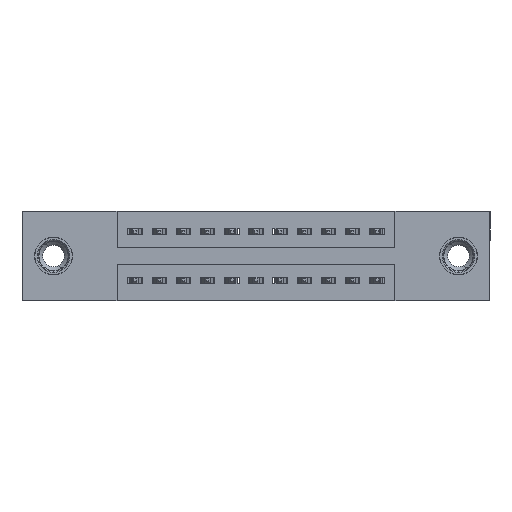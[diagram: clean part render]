
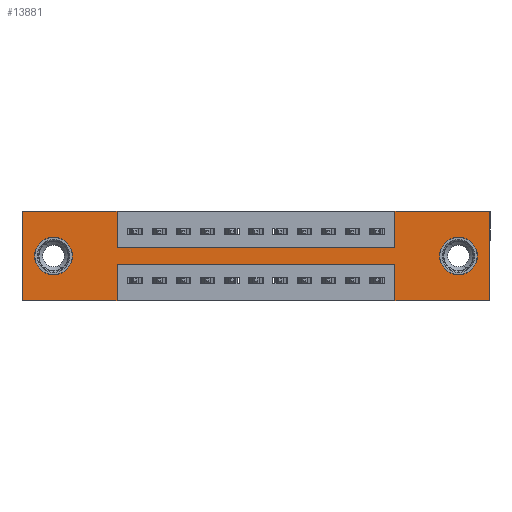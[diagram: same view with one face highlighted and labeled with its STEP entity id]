
A CAD part, front view. The second image highlights one B-rep face of the part: STEP entity #13881.
In plain terms, the highlighted planar face has unit normal (0, -1, 0).
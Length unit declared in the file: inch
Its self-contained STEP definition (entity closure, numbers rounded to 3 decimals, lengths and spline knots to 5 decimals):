
#4 = DIRECTION ( 'NONE',  ( 0., 0., -1. ) ) ;
#29 = CARTESIAN_POINT ( 'NONE',  ( 1.5425, 0., 0. ) ) ;
#186 = EDGE_CURVE ( 'NONE', #11152, #595, #14252, .T. ) ;
#595 = VERTEX_POINT ( 'NONE', #15899 ) ;
#646 = CIRCLE ( 'NONE', #2475, 0.078 ) ;
#793 = AXIS2_PLACEMENT_3D ( 'NONE', #12753, #14285, #6076 ) ;
#917 = CIRCLE ( 'NONE', #13022, 0.078 ) ;
#1027 = ORIENTED_EDGE ( 'NONE', *, *, #2276, .F. ) ;
#1037 = CARTESIAN_POINT ( 'NONE',  ( 0., 0., -0.37 ) ) ;
#1091 = DIRECTION ( 'NONE',  ( 0., -1., 0. ) ) ;
#1112 = EDGE_CURVE ( 'NONE', #6410, #12176, #646, .T. ) ;
#1217 = VERTEX_POINT ( 'NONE', #5519 ) ;
#1307 = DIRECTION ( 'NONE',  ( -1., 0., 0. ) ) ;
#1494 = ORIENTED_EDGE ( 'NONE', *, *, #11015, .F. ) ;
#1873 = EDGE_CURVE ( 'NONE', #595, #14750, #13383, .T. ) ;
#1982 = CARTESIAN_POINT ( 'NONE',  ( 0., 0., -0.37 ) ) ;
#2038 = DIRECTION ( 'NONE',  ( 0., 1., 0. ) ) ;
#2178 = FACE_BOUND ( 'NONE', #6233, .T. ) ;
#2208 = VERTEX_POINT ( 'NONE', #7370 ) ;
#2276 = EDGE_CURVE ( 'NONE', #14750, #14485, #16325, .T. ) ;
#2378 = LINE ( 'NONE', #16224, #17463 ) ;
#2394 = EDGE_LOOP ( 'NONE', ( #10713, #16401 ) ) ;
#2475 = AXIS2_PLACEMENT_3D ( 'NONE', #17480, #9263, #9315 ) ;
#2486 = ORIENTED_EDGE ( 'NONE', *, *, #6051, .T. ) ;
#2535 = VECTOR ( 'NONE', #13410, 39.37008 ) ;
#2538 = CARTESIAN_POINT ( 'NONE',  ( 0., 0., -0.37 ) ) ;
#2643 = ORIENTED_EDGE ( 'NONE', *, *, #10460, .F. ) ;
#2704 = VECTOR ( 'NONE', #10745, 39.37008 ) ;
#3094 = LINE ( 'NONE', #14840, #7967 ) ;
#3532 = VERTEX_POINT ( 'NONE', #29 ) ;
#3795 = DIRECTION ( 'NONE',  ( 0., 0., -1. ) ) ;
#3907 = DIRECTION ( 'NONE',  ( 0., 0., -1. ) ) ;
#3909 = EDGE_CURVE ( 'NONE', #1217, #11836, #12257, .T. ) ;
#3942 = AXIS2_PLACEMENT_3D ( 'NONE', #1037, #1091, #3795 ) ;
#4038 = EDGE_CURVE ( 'NONE', #14485, #5997, #5833, .T. ) ;
#4094 = PLANE ( 'NONE',  #3942 ) ;
#4148 = CARTESIAN_POINT ( 'NONE',  ( 0.3925, 0., 0. ) ) ;
#4479 = DIRECTION ( 'NONE',  ( 1., 0., 0. ) ) ;
#4730 = ORIENTED_EDGE ( 'NONE', *, *, #4038, .F. ) ;
#4836 = LINE ( 'NONE', #4148, #9075 ) ;
#5200 = ORIENTED_EDGE ( 'NONE', *, *, #15772, .F. ) ;
#5343 = LINE ( 'NONE', #12643, #8520 ) ;
#5519 = CARTESIAN_POINT ( 'NONE',  ( 0.3925, 0., -0.37 ) ) ;
#5765 = FACE_BOUND ( 'NONE', #2394, .T. ) ;
#5833 = LINE ( 'NONE', #6760, #15400 ) ;
#5997 = VERTEX_POINT ( 'NONE', #7391 ) ;
#6051 = EDGE_CURVE ( 'NONE', #12176, #6410, #9373, .T. ) ;
#6076 = DIRECTION ( 'NONE',  ( 0., 0., -1. ) ) ;
#6093 = LINE ( 'NONE', #13523, #2704 ) ;
#6233 = EDGE_LOOP ( 'NONE', ( #2486, #9530 ) ) ;
#6410 = VERTEX_POINT ( 'NONE', #8038 ) ;
#6420 = EDGE_CURVE ( 'NONE', #9613, #2208, #917, .T. ) ;
#6482 = ORIENTED_EDGE ( 'NONE', *, *, #3909, .F. ) ;
#6563 = EDGE_CURVE ( 'NONE', #11707, #15622, #5343, .T. ) ;
#6593 = CARTESIAN_POINT ( 'NONE',  ( 1.5425, 0., -0.37 ) ) ;
#6622 = FACE_OUTER_BOUND ( 'NONE', #13004, .T. ) ;
#6669 = EDGE_CURVE ( 'NONE', #5997, #1217, #10465, .T. ) ;
#6712 = DIRECTION ( 'NONE',  ( 0., 0., 1. ) ) ;
#6760 = CARTESIAN_POINT ( 'NONE',  ( 0.3925, 0., -0.22 ) ) ;
#7326 = DIRECTION ( 'NONE',  ( 1., 0., 0. ) ) ;
#7370 = CARTESIAN_POINT ( 'NONE',  ( 1.805, 0., -0.263 ) ) ;
#7391 = CARTESIAN_POINT ( 'NONE',  ( 0.3925, 0., -0.22 ) ) ;
#7558 = ORIENTED_EDGE ( 'NONE', *, *, #186, .F. ) ;
#7594 = EDGE_CURVE ( 'NONE', #13691, #3532, #2378, .T. ) ;
#7871 = VERTEX_POINT ( 'NONE', #12721 ) ;
#7967 = VECTOR ( 'NONE', #12130, 39.37008 ) ;
#8038 = CARTESIAN_POINT ( 'NONE',  ( 0.13, 0., -0.263 ) ) ;
#8065 = CARTESIAN_POINT ( 'NONE',  ( 0., 0., 0. ) ) ;
#8520 = VECTOR ( 'NONE', #4479, 39.37008 ) ;
#9075 = VECTOR ( 'NONE', #3907, 39.37008 ) ;
#9263 = DIRECTION ( 'NONE',  ( 0., 1., 0. ) ) ;
#9315 = DIRECTION ( 'NONE',  ( 0., 0., 1. ) ) ;
#9373 = CIRCLE ( 'NONE', #11655, 0.078 ) ;
#9530 = ORIENTED_EDGE ( 'NONE', *, *, #1112, .T. ) ;
#9613 = VERTEX_POINT ( 'NONE', #10181 ) ;
#9660 = ORIENTED_EDGE ( 'NONE', *, *, #6669, .F. ) ;
#10110 = VECTOR ( 'NONE', #7326, 39.37008 ) ;
#10181 = CARTESIAN_POINT ( 'NONE',  ( 1.805, 0., -0.107 ) ) ;
#10186 = CARTESIAN_POINT ( 'NONE',  ( 1.5425, 0., -0.37 ) ) ;
#10460 = EDGE_CURVE ( 'NONE', #15622, #7871, #4836, .T. ) ;
#10465 = LINE ( 'NONE', #12815, #13217 ) ;
#10713 = ORIENTED_EDGE ( 'NONE', *, *, #6420, .T. ) ;
#10745 = DIRECTION ( 'NONE',  ( 1., 0., 0. ) ) ;
#10813 = DIRECTION ( 'NONE',  ( 0., 1., 0. ) ) ;
#11004 = CARTESIAN_POINT ( 'NONE',  ( 0.13, 0., -0.107 ) ) ;
#11015 = EDGE_CURVE ( 'NONE', #3532, #11152, #6093, .T. ) ;
#11152 = VERTEX_POINT ( 'NONE', #16601 ) ;
#11471 = DIRECTION ( 'NONE',  ( 0., 0., 1. ) ) ;
#11655 = AXIS2_PLACEMENT_3D ( 'NONE', #12836, #2038, #11471 ) ;
#11707 = VERTEX_POINT ( 'NONE', #8065 ) ;
#11836 = VERTEX_POINT ( 'NONE', #1982 ) ;
#12130 = DIRECTION ( 'NONE',  ( 0., 0., 1. ) ) ;
#12176 = VERTEX_POINT ( 'NONE', #11004 ) ;
#12257 = LINE ( 'NONE', #15982, #16069 ) ;
#12643 = CARTESIAN_POINT ( 'NONE',  ( 0., 0., 0. ) ) ;
#12721 = CARTESIAN_POINT ( 'NONE',  ( 0.3925, 0., -0.15 ) ) ;
#12753 = CARTESIAN_POINT ( 'NONE',  ( 1.805, 0., -0.185 ) ) ;
#12815 = CARTESIAN_POINT ( 'NONE',  ( 0.3925, 0., -0.37 ) ) ;
#12836 = CARTESIAN_POINT ( 'NONE',  ( 0.13, 0., -0.185 ) ) ;
#13004 = EDGE_LOOP ( 'NONE', ( #9660, #4730, #1027, #15089, #7558, #1494, #17531, #15372, #2643, #13576, #5200, #6482 ) ) ;
#13022 = AXIS2_PLACEMENT_3D ( 'NONE', #15015, #10813, #4 ) ;
#13217 = VECTOR ( 'NONE', #15654, 39.37008 ) ;
#13301 = CARTESIAN_POINT ( 'NONE',  ( 1.5425, 0., -0.22 ) ) ;
#13383 = LINE ( 'NONE', #2538, #2535 ) ;
#13410 = DIRECTION ( 'NONE',  ( -1., 0., 0. ) ) ;
#13467 = DIRECTION ( 'NONE',  ( 0., 0., -1. ) ) ;
#13523 = CARTESIAN_POINT ( 'NONE',  ( 0., 0., 0. ) ) ;
#13576 = ORIENTED_EDGE ( 'NONE', *, *, #6563, .F. ) ;
#13691 = VERTEX_POINT ( 'NONE', #16883 ) ;
#13881 = ADVANCED_FACE ( 'NONE', ( #5765, #2178, #6622 ), #4094, .T. ) ;
#14252 = LINE ( 'NONE', #15236, #14668 ) ;
#14285 = DIRECTION ( 'NONE',  ( 0., 1., 0. ) ) ;
#14485 = VERTEX_POINT ( 'NONE', #13301 ) ;
#14498 = DIRECTION ( 'NONE',  ( -1., 0., 0. ) ) ;
#14668 = VECTOR ( 'NONE', #13467, 39.37008 ) ;
#14721 = EDGE_CURVE ( 'NONE', #2208, #9613, #17385, .T. ) ;
#14750 = VERTEX_POINT ( 'NONE', #10186 ) ;
#14777 = LINE ( 'NONE', #15482, #10110 ) ;
#14840 = CARTESIAN_POINT ( 'NONE',  ( 0., 0., 0. ) ) ;
#14979 = DIRECTION ( 'NONE',  ( 0., 0., 1. ) ) ;
#15015 = CARTESIAN_POINT ( 'NONE',  ( 1.805, 0., -0.185 ) ) ;
#15089 = ORIENTED_EDGE ( 'NONE', *, *, #1873, .F. ) ;
#15236 = CARTESIAN_POINT ( 'NONE',  ( 1.935, 0., 0. ) ) ;
#15372 = ORIENTED_EDGE ( 'NONE', *, *, #16060, .F. ) ;
#15400 = VECTOR ( 'NONE', #1307, 39.37008 ) ;
#15482 = CARTESIAN_POINT ( 'NONE',  ( 0.3925, 0., -0.15 ) ) ;
#15622 = VERTEX_POINT ( 'NONE', #15812 ) ;
#15654 = DIRECTION ( 'NONE',  ( 0., 0., -1. ) ) ;
#15772 = EDGE_CURVE ( 'NONE', #11836, #11707, #3094, .T. ) ;
#15812 = CARTESIAN_POINT ( 'NONE',  ( 0.3925, 0., 0. ) ) ;
#15899 = CARTESIAN_POINT ( 'NONE',  ( 1.935, 0., -0.37 ) ) ;
#15982 = CARTESIAN_POINT ( 'NONE',  ( 0., 0., -0.37 ) ) ;
#16060 = EDGE_CURVE ( 'NONE', #7871, #13691, #14777, .T. ) ;
#16069 = VECTOR ( 'NONE', #14498, 39.37008 ) ;
#16224 = CARTESIAN_POINT ( 'NONE',  ( 1.5425, 0., 0. ) ) ;
#16325 = LINE ( 'NONE', #6593, #16967 ) ;
#16401 = ORIENTED_EDGE ( 'NONE', *, *, #14721, .T. ) ;
#16601 = CARTESIAN_POINT ( 'NONE',  ( 1.935, 0., 0. ) ) ;
#16883 = CARTESIAN_POINT ( 'NONE',  ( 1.5425, 0., -0.15 ) ) ;
#16967 = VECTOR ( 'NONE', #6712, 39.37008 ) ;
#17385 = CIRCLE ( 'NONE', #793, 0.078 ) ;
#17463 = VECTOR ( 'NONE', #14979, 39.37008 ) ;
#17480 = CARTESIAN_POINT ( 'NONE',  ( 0.13, 0., -0.185 ) ) ;
#17531 = ORIENTED_EDGE ( 'NONE', *, *, #7594, .F. ) ;
